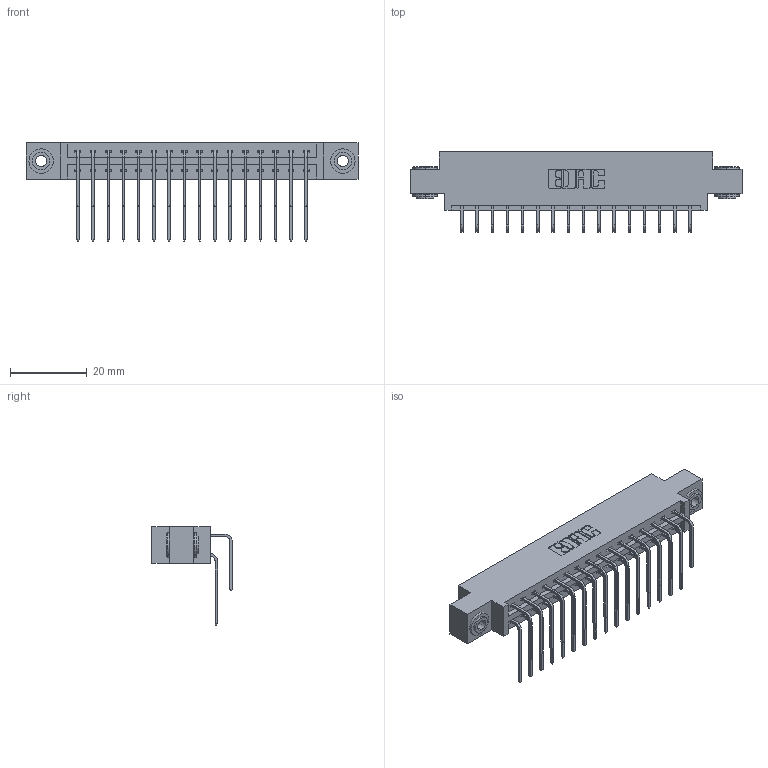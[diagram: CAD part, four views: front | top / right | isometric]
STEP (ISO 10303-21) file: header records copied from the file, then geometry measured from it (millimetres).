
FILE_DESCRIPTION (( 'STEP AP203' ), '1' );
FILE_NAME ('337-032-559-803.STEP', '2019-10-11T01:17:33', ( '' ), ( '' ), 'SwSTEP 2.0', 'SolidWorks 2016', '' );
FILE_SCHEMA (( 'CONFIG_CONTROL_DESIGN' ));
Length unit declared in the file: inch
Products named in the file (5): 337 Part_0.170 Offset - 0.156 Dia-TH; 345-292-001_559 Tail - 2; 345-292-001_558 559 Tail - 1; 337-032-559-803; 345-250-002_345-250-002-102
Assembly tree (35 placements, depth 2):
  337-032-559-803
    337 Part_0.170 Offset - 0.156 Dia-TH
    345-292-001_558 559 Tail - 1  x16
    345-292-001_559 Tail - 2  x16
    345-250-002_345-250-002-102  x2
Bounding box: 86.41 x 20.9 x 25.53 mm (x, y, z)
Volume: 8847.1 mm3; surface area: 11008.2 mm2
Topology: 35 solids, 35 shells, 1948 faces, 5743 edges, 3782 vertices
Faces by surface type: plane 1364, cylinder 576, cone 8
Entity records: 18334 total; most frequent: CARTESIAN_POINT 3132, ORIENTED_EDGE 3010, DIRECTION 2727, EDGE_CURVE 1505, LINE 1313, VECTOR 1313, VERTEX_POINT 998, AXIS2_PLACEMENT_3D 707
